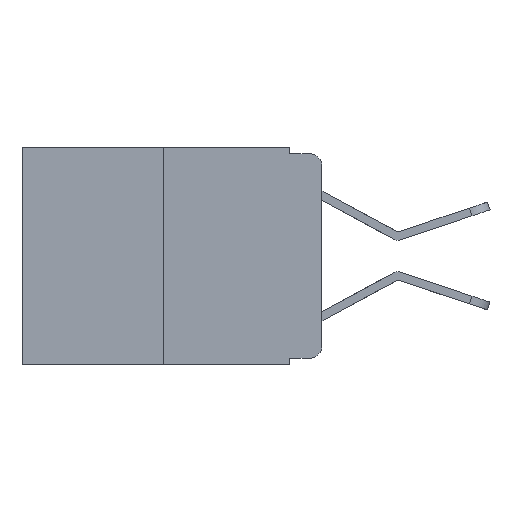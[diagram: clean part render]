
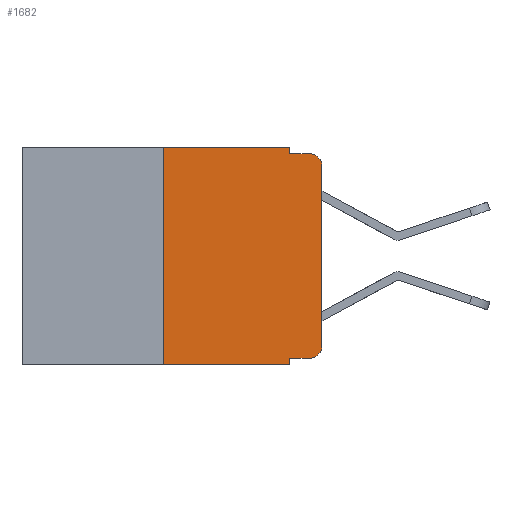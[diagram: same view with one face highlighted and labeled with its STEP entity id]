
A CAD part, left-side view. The second image highlights one B-rep face of the part: STEP entity #1682.
In plain terms, the highlighted planar face has unit normal (-1, 0, 0).
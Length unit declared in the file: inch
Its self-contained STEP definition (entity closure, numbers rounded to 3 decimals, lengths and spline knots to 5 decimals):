
#290 = CARTESIAN_POINT ( 'NONE',  ( 0., 0., 0. ) ) ;
#1069 = DIRECTION ( 'NONE',  ( 0., -1., 0. ) ) ;
#1321 = LINE ( 'NONE', #2958, #11110 ) ;
#1379 = LINE ( 'NONE', #290, #15631 ) ;
#1486 = CARTESIAN_POINT ( 'NONE',  ( 0., 0.473, 0. ) ) ;
#1563 = DIRECTION ( 'NONE',  ( 0., -1., 0. ) ) ;
#1629 = CARTESIAN_POINT ( 'NONE',  ( 0., 0.25, 0. ) ) ;
#1682 = ADVANCED_FACE ( 'NONE', ( #5580 ), #18542, .F. ) ;
#1885 = DIRECTION ( 'NONE',  ( 0., -1., 0. ) ) ;
#2040 = CARTESIAN_POINT ( 'NONE',  ( 0., 0.051, 0. ) ) ;
#2137 = VERTEX_POINT ( 'NONE', #15672 ) ;
#2142 = LINE ( 'NONE', #24231, #5411 ) ;
#2186 = EDGE_CURVE ( 'NONE', #2137, #5546, #16528, .T. ) ;
#2396 = CARTESIAN_POINT ( 'NONE',  ( 0., 0.02, -0.01 ) ) ;
#2572 = LINE ( 'NONE', #13235, #20699 ) ;
#2958 = CARTESIAN_POINT ( 'NONE',  ( 0., 0.051, 0. ) ) ;
#3451 = DIRECTION ( 'NONE',  ( 1., 0., 0. ) ) ;
#4517 = EDGE_CURVE ( 'NONE', #11877, #12248, #21822, .T. ) ;
#4726 = AXIS2_PLACEMENT_3D ( 'NONE', #14974, #3451, #18620 ) ;
#5271 = CARTESIAN_POINT ( 'NONE',  ( 0., 0., -0.03 ) ) ;
#5294 = CARTESIAN_POINT ( 'NONE',  ( 0., 0.02, -0.313 ) ) ;
#5411 = VECTOR ( 'NONE', #7249, 39.37008 ) ;
#5546 = VERTEX_POINT ( 'NONE', #2396 ) ;
#5580 = FACE_OUTER_BOUND ( 'NONE', #6759, .T. ) ;
#6698 = DIRECTION ( 'NONE',  ( 0., 0., -1. ) ) ;
#6707 = CARTESIAN_POINT ( 'NONE',  ( 0., 0.051, -0.343 ) ) ;
#6759 = EDGE_LOOP ( 'NONE', ( #11315, #13416, #7362, #20792, #14553, #21168, #6908, #8017, #19320, #9011 ) ) ;
#6908 = ORIENTED_EDGE ( 'NONE', *, *, #19684, .T. ) ;
#7095 = CIRCLE ( 'NONE', #16252, 0.02 ) ;
#7249 = DIRECTION ( 'NONE',  ( 0., -1., 0. ) ) ;
#7362 = ORIENTED_EDGE ( 'NONE', *, *, #2186, .F. ) ;
#7520 = EDGE_CURVE ( 'NONE', #14905, #23665, #7095, .T. ) ;
#7692 = VERTEX_POINT ( 'NONE', #2040 ) ;
#7823 = CARTESIAN_POINT ( 'NONE',  ( 0., 0., -0.313 ) ) ;
#8017 = ORIENTED_EDGE ( 'NONE', *, *, #10012, .F. ) ;
#9011 = ORIENTED_EDGE ( 'NONE', *, *, #7520, .T. ) ;
#9094 = DIRECTION ( 'NONE',  ( -1., 0., 0. ) ) ;
#9141 = CARTESIAN_POINT ( 'NONE',  ( 0., 0.051, -0.333 ) ) ;
#9628 = AXIS2_PLACEMENT_3D ( 'NONE', #15128, #18943, #11447 ) ;
#10012 = EDGE_CURVE ( 'NONE', #10915, #18707, #1321, .T. ) ;
#10423 = CARTESIAN_POINT ( 'NONE',  ( 0., 0.051, 0. ) ) ;
#10915 = VERTEX_POINT ( 'NONE', #9141 ) ;
#11110 = VECTOR ( 'NONE', #20211, 39.37008 ) ;
#11315 = ORIENTED_EDGE ( 'NONE', *, *, #23590, .T. ) ;
#11447 = DIRECTION ( 'NONE',  ( 0., 0., -1. ) ) ;
#11460 = EDGE_CURVE ( 'NONE', #10915, #14905, #2572, .T. ) ;
#11877 = VERTEX_POINT ( 'NONE', #22464 ) ;
#12248 = VERTEX_POINT ( 'NONE', #18576 ) ;
#12408 = CARTESIAN_POINT ( 'NONE',  ( 0., 0.051, -0.01 ) ) ;
#13235 = CARTESIAN_POINT ( 'NONE',  ( 0., 0.051, -0.333 ) ) ;
#13393 = VERTEX_POINT ( 'NONE', #5271 ) ;
#13416 = ORIENTED_EDGE ( 'NONE', *, *, #16070, .T. ) ;
#13832 = VECTOR ( 'NONE', #1069, 39.37008 ) ;
#14553 = ORIENTED_EDGE ( 'NONE', *, *, #18832, .F. ) ;
#14635 = DIRECTION ( 'NONE',  ( 0., 0., 1. ) ) ;
#14905 = VERTEX_POINT ( 'NONE', #21269 ) ;
#14974 = CARTESIAN_POINT ( 'NONE',  ( 0., 0.473, 0. ) ) ;
#14975 = LINE ( 'NONE', #1486, #18227 ) ;
#15126 = EDGE_CURVE ( 'NONE', #7692, #2137, #20533, .T. ) ;
#15128 = CARTESIAN_POINT ( 'NONE',  ( 0., 0.02, -0.03 ) ) ;
#15631 = VECTOR ( 'NONE', #19165, 39.37008 ) ;
#15672 = CARTESIAN_POINT ( 'NONE',  ( 0., 0.051, -0.01 ) ) ;
#16070 = EDGE_CURVE ( 'NONE', #13393, #5546, #20198, .T. ) ;
#16252 = AXIS2_PLACEMENT_3D ( 'NONE', #5294, #9094, #22268 ) ;
#16528 = LINE ( 'NONE', #12408, #13832 ) ;
#16763 = VECTOR ( 'NONE', #14635, 39.37008 ) ;
#18227 = VECTOR ( 'NONE', #1563, 39.37008 ) ;
#18542 = PLANE ( 'NONE',  #4726 ) ;
#18576 = CARTESIAN_POINT ( 'NONE',  ( 0., 0.25, 0. ) ) ;
#18620 = DIRECTION ( 'NONE',  ( 0., 0., -1. ) ) ;
#18707 = VERTEX_POINT ( 'NONE', #6707 ) ;
#18832 = EDGE_CURVE ( 'NONE', #12248, #7692, #14975, .T. ) ;
#18943 = DIRECTION ( 'NONE',  ( -1., 0., 0. ) ) ;
#19165 = DIRECTION ( 'NONE',  ( 0., 0., 1. ) ) ;
#19320 = ORIENTED_EDGE ( 'NONE', *, *, #11460, .T. ) ;
#19684 = EDGE_CURVE ( 'NONE', #11877, #18707, #2142, .T. ) ;
#20198 = CIRCLE ( 'NONE', #9628, 0.02 ) ;
#20211 = DIRECTION ( 'NONE',  ( 0., 0., -1. ) ) ;
#20533 = LINE ( 'NONE', #10423, #23761 ) ;
#20699 = VECTOR ( 'NONE', #1885, 39.37008 ) ;
#20792 = ORIENTED_EDGE ( 'NONE', *, *, #15126, .F. ) ;
#21168 = ORIENTED_EDGE ( 'NONE', *, *, #4517, .F. ) ;
#21269 = CARTESIAN_POINT ( 'NONE',  ( 0., 0.02, -0.333 ) ) ;
#21822 = LINE ( 'NONE', #1629, #16763 ) ;
#22268 = DIRECTION ( 'NONE',  ( 0., 0., -1. ) ) ;
#22464 = CARTESIAN_POINT ( 'NONE',  ( 0., 0.25, -0.343 ) ) ;
#23590 = EDGE_CURVE ( 'NONE', #23665, #13393, #1379, .T. ) ;
#23665 = VERTEX_POINT ( 'NONE', #7823 ) ;
#23761 = VECTOR ( 'NONE', #6698, 39.37008 ) ;
#24231 = CARTESIAN_POINT ( 'NONE',  ( 0., 0.473, -0.343 ) ) ;
